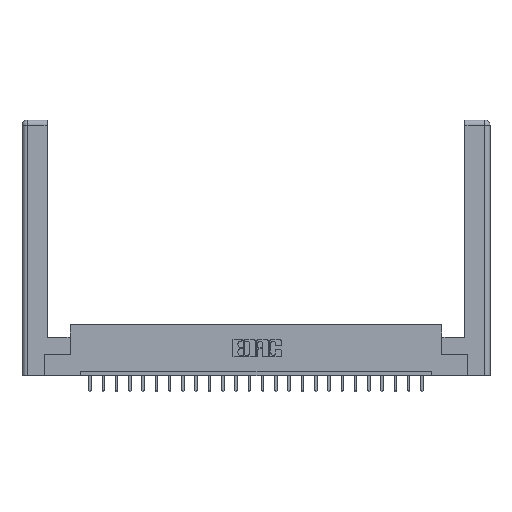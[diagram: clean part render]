
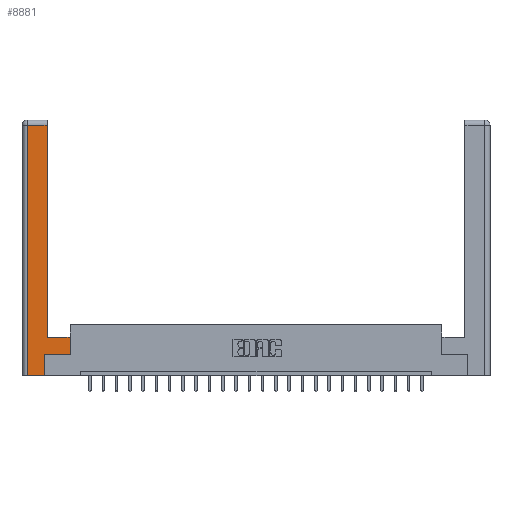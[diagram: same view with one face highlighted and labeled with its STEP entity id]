
A CAD part, top view. The second image highlights one B-rep face of the part: STEP entity #8881.
In plain terms, the highlighted planar face has unit normal (0, 0, 1).
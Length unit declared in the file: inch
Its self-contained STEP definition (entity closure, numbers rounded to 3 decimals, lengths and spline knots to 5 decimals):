
#406 = CARTESIAN_POINT ( 'NONE',  ( 0.295, 0.45, 0. ) ) ;
#741 = PLANE ( 'NONE',  #21483 ) ;
#1007 = VERTEX_POINT ( 'NONE', #14871 ) ;
#1465 = CARTESIAN_POINT ( 'NONE',  ( 0.565, 0.245, 0. ) ) ;
#1653 = DIRECTION ( 'NONE',  ( 1., 0., 0. ) ) ;
#1929 = VERTEX_POINT ( 'NONE', #3285 ) ;
#2312 = CARTESIAN_POINT ( 'NONE',  ( 0., 0., 0. ) ) ;
#2620 = DIRECTION ( 'NONE',  ( 1., 0., 0. ) ) ;
#2744 = CARTESIAN_POINT ( 'NONE',  ( 0.565, 0.45, 0. ) ) ;
#3285 = CARTESIAN_POINT ( 'NONE',  ( 0.0615, 0., 0. ) ) ;
#3330 = VECTOR ( 'NONE', #14754, 39.37008 ) ;
#3424 = CARTESIAN_POINT ( 'NONE',  ( 0.565, 0.45, 0. ) ) ;
#3508 = DIRECTION ( 'NONE',  ( 0., 1., 0. ) ) ;
#3688 = ORIENTED_EDGE ( 'NONE', *, *, #12883, .T. ) ;
#3756 = ORIENTED_EDGE ( 'NONE', *, *, #14477, .T. ) ;
#3759 = VECTOR ( 'NONE', #17399, 39.37008 ) ;
#4449 = LINE ( 'NONE', #2744, #8830 ) ;
#4767 = LINE ( 'NONE', #9070, #3330 ) ;
#5105 = FACE_OUTER_BOUND ( 'NONE', #7423, .T. ) ;
#5327 = VERTEX_POINT ( 'NONE', #3424 ) ;
#5958 = EDGE_CURVE ( 'NONE', #1929, #1007, #15728, .T. ) ;
#6145 = DIRECTION ( 'NONE',  ( 0., 0., -1. ) ) ;
#6407 = DIRECTION ( 'NONE',  ( 0., 1., 0. ) ) ;
#6652 = VERTEX_POINT ( 'NONE', #10568 ) ;
#7333 = ORIENTED_EDGE ( 'NONE', *, *, #23886, .T. ) ;
#7423 = EDGE_LOOP ( 'NONE', ( #3756, #3688, #7333, #10937, #22500, #21647, #13021, #11440 ) ) ;
#7727 = VERTEX_POINT ( 'NONE', #12375 ) ;
#7984 = CARTESIAN_POINT ( 'NONE',  ( 0.0615, 2.94, 0. ) ) ;
#8191 = DIRECTION ( 'NONE',  ( -1., 0., 0. ) ) ;
#8830 = VECTOR ( 'NONE', #6407, 39.37008 ) ;
#8881 = ADVANCED_FACE ( 'NONE', ( #5105 ), #741, .F. ) ;
#9070 = CARTESIAN_POINT ( 'NONE',  ( 0.295, 3., 0. ) ) ;
#9244 = VECTOR ( 'NONE', #18923, 39.37008 ) ;
#9819 = EDGE_CURVE ( 'NONE', #12958, #11341, #18802, .T. ) ;
#10568 = CARTESIAN_POINT ( 'NONE',  ( 0.295, 2.94, 0. ) ) ;
#10877 = CARTESIAN_POINT ( 'NONE',  ( 0.265, 0., 0. ) ) ;
#10937 = ORIENTED_EDGE ( 'NONE', *, *, #5958, .T. ) ;
#11060 = EDGE_CURVE ( 'NONE', #5327, #14116, #16597, .T. ) ;
#11341 = VERTEX_POINT ( 'NONE', #1465 ) ;
#11440 = ORIENTED_EDGE ( 'NONE', *, *, #11060, .T. ) ;
#11769 = CARTESIAN_POINT ( 'NONE',  ( 0.295, 0.45, 0. ) ) ;
#12375 = CARTESIAN_POINT ( 'NONE',  ( 0.0615, 2.94, 0. ) ) ;
#12883 = EDGE_CURVE ( 'NONE', #6652, #7727, #22355, .T. ) ;
#12958 = VERTEX_POINT ( 'NONE', #19490 ) ;
#13021 = ORIENTED_EDGE ( 'NONE', *, *, #18187, .T. ) ;
#13795 = VECTOR ( 'NONE', #2620, 39.37008 ) ;
#14116 = VERTEX_POINT ( 'NONE', #406 ) ;
#14477 = EDGE_CURVE ( 'NONE', #14116, #6652, #4767, .T. ) ;
#14645 = CARTESIAN_POINT ( 'NONE',  ( 0.265, 0.245, 0. ) ) ;
#14754 = DIRECTION ( 'NONE',  ( 0., 1., 0. ) ) ;
#14871 = CARTESIAN_POINT ( 'NONE',  ( 0.265, 0., 0. ) ) ;
#15728 = LINE ( 'NONE', #10877, #19310 ) ;
#16597 = LINE ( 'NONE', #11769, #3759 ) ;
#17058 = LINE ( 'NONE', #21497, #18527 ) ;
#17399 = DIRECTION ( 'NONE',  ( -1., 0., 0. ) ) ;
#17602 = LINE ( 'NONE', #14645, #21403 ) ;
#17856 = EDGE_CURVE ( 'NONE', #1007, #12958, #17602, .T. ) ;
#18187 = EDGE_CURVE ( 'NONE', #11341, #5327, #4449, .T. ) ;
#18527 = VECTOR ( 'NONE', #19456, 39.37008 ) ;
#18802 = LINE ( 'NONE', #23067, #13795 ) ;
#18923 = DIRECTION ( 'NONE',  ( -1., 0., 0. ) ) ;
#19310 = VECTOR ( 'NONE', #1653, 39.37008 ) ;
#19456 = DIRECTION ( 'NONE',  ( 0., -1., 0. ) ) ;
#19490 = CARTESIAN_POINT ( 'NONE',  ( 0.265, 0.245, 0. ) ) ;
#21403 = VECTOR ( 'NONE', #3508, 39.37008 ) ;
#21483 = AXIS2_PLACEMENT_3D ( 'NONE', #2312, #6145, #8191 ) ;
#21497 = CARTESIAN_POINT ( 'NONE',  ( 0.0615, 0., 0. ) ) ;
#21647 = ORIENTED_EDGE ( 'NONE', *, *, #9819, .T. ) ;
#22355 = LINE ( 'NONE', #7984, #9244 ) ;
#22500 = ORIENTED_EDGE ( 'NONE', *, *, #17856, .T. ) ;
#23067 = CARTESIAN_POINT ( 'NONE',  ( 0.565, 0.245, 0. ) ) ;
#23886 = EDGE_CURVE ( 'NONE', #7727, #1929, #17058, .T. ) ;
